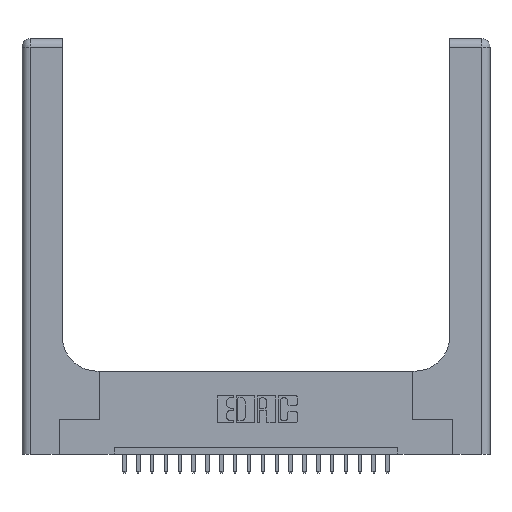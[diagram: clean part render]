
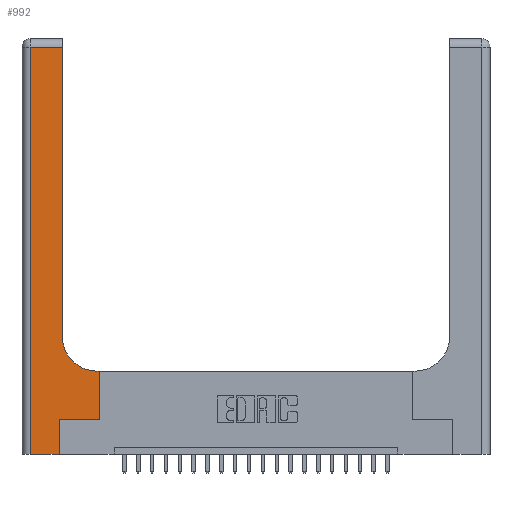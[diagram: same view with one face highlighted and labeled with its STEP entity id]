
A CAD part, top view. The second image highlights one B-rep face of the part: STEP entity #992.
In plain terms, the highlighted planar face has unit normal (0, 0, 1).
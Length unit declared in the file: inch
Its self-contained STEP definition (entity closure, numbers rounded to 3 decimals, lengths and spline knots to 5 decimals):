
#124 = LINE ( 'NONE', #13736, #7437 ) ;
#361 = ORIENTED_EDGE ( 'NONE', *, *, #13297, .T. ) ;
#371 = EDGE_CURVE ( 'NONE', #22887, #6382, #17491, .T. ) ;
#621 = CARTESIAN_POINT ( 'NONE',  ( 0.5585, 0.6, 0.37 ) ) ;
#992 = ADVANCED_FACE ( 'NONE', ( #4005 ), #1167, .F. ) ;
#1020 = EDGE_CURVE ( 'NONE', #8691, #11430, #9333, .T. ) ;
#1040 = DIRECTION ( 'NONE',  ( -1., 0., 0. ) ) ;
#1042 = CARTESIAN_POINT ( 'NONE',  ( 0.269, 0.25, 0.37 ) ) ;
#1167 = PLANE ( 'NONE',  #19967 ) ;
#1243 = VECTOR ( 'NONE', #13216, 39.37008 ) ;
#1485 = CARTESIAN_POINT ( 'NONE',  ( 0.5585, 0.25, 0.37 ) ) ;
#1492 = VECTOR ( 'NONE', #1040, 39.37008 ) ;
#1507 = DIRECTION ( 'NONE',  ( 0., 1., 0. ) ) ;
#1599 = EDGE_CURVE ( 'NONE', #6382, #12002, #2591, .T. ) ;
#1628 = VERTEX_POINT ( 'NONE', #5102 ) ;
#1868 = ORIENTED_EDGE ( 'NONE', *, *, #1020, .T. ) ;
#2591 = LINE ( 'NONE', #19506, #10448 ) ;
#3507 = CARTESIAN_POINT ( 'NONE',  ( 0.5415, 0.85, 0.37 ) ) ;
#4005 = FACE_OUTER_BOUND ( 'NONE', #4035, .T. ) ;
#4035 = EDGE_LOOP ( 'NONE', ( #21562, #4412, #14069, #1868, #361, #22215, #22430, #14792, #4625 ) ) ;
#4412 = ORIENTED_EDGE ( 'NONE', *, *, #15779, .T. ) ;
#4625 = ORIENTED_EDGE ( 'NONE', *, *, #12487, .T. ) ;
#4893 = LINE ( 'NONE', #6259, #1243 ) ;
#5102 = CARTESIAN_POINT ( 'NONE',  ( 0.5415, 0.6, 0.37 ) ) ;
#5917 = LINE ( 'NONE', #19730, #7877 ) ;
#6007 = VECTOR ( 'NONE', #8025, 39.37008 ) ;
#6259 = CARTESIAN_POINT ( 'NONE',  ( 0.269, 0., 0.37 ) ) ;
#6382 = VERTEX_POINT ( 'NONE', #1485 ) ;
#6925 = CIRCLE ( 'NONE', #10398, 0.25 ) ;
#7065 = VERTEX_POINT ( 'NONE', #12906 ) ;
#7305 = CARTESIAN_POINT ( 'NONE',  ( 0.269, 0., 0.37 ) ) ;
#7437 = VECTOR ( 'NONE', #1507, 39.37008 ) ;
#7480 = DIRECTION ( 'NONE',  ( 1., 0., 0. ) ) ;
#7866 = VERTEX_POINT ( 'NONE', #12911 ) ;
#7877 = VECTOR ( 'NONE', #16225, 39.37008 ) ;
#8025 = DIRECTION ( 'NONE',  ( 1., 0., 0. ) ) ;
#8691 = VERTEX_POINT ( 'NONE', #17017 ) ;
#9333 = LINE ( 'NONE', #12786, #12972 ) ;
#9753 = CARTESIAN_POINT ( 'NONE',  ( 0.269, 0.25, 0.37 ) ) ;
#10398 = AXIS2_PLACEMENT_3D ( 'NONE', #3507, #23228, #10555 ) ;
#10448 = VECTOR ( 'NONE', #23183, 39.37008 ) ;
#10555 = DIRECTION ( 'NONE',  ( 1., 0., 0. ) ) ;
#11430 = VERTEX_POINT ( 'NONE', #7305 ) ;
#12002 = VERTEX_POINT ( 'NONE', #621 ) ;
#12487 = EDGE_CURVE ( 'NONE', #1628, #7866, #6925, .T. ) ;
#12786 = CARTESIAN_POINT ( 'NONE',  ( 0., 0., 0.37 ) ) ;
#12906 = CARTESIAN_POINT ( 'NONE',  ( 0.2915, 2.94, 0.37 ) ) ;
#12911 = CARTESIAN_POINT ( 'NONE',  ( 0.2915, 0.85, 0.37 ) ) ;
#12972 = VECTOR ( 'NONE', #7480, 39.37008 ) ;
#13191 = LINE ( 'NONE', #21080, #15462 ) ;
#13216 = DIRECTION ( 'NONE',  ( 0., 1., 0. ) ) ;
#13297 = EDGE_CURVE ( 'NONE', #11430, #22887, #4893, .T. ) ;
#13736 = CARTESIAN_POINT ( 'NONE',  ( 0.2915, 3., 0.37 ) ) ;
#13874 = EDGE_CURVE ( 'NONE', #12002, #1628, #21921, .T. ) ;
#13980 = CARTESIAN_POINT ( 'NONE',  ( 0.06, 2.94, 0.37 ) ) ;
#14069 = ORIENTED_EDGE ( 'NONE', *, *, #16482, .T. ) ;
#14213 = DIRECTION ( 'NONE',  ( -1., 0., 0. ) ) ;
#14698 = DIRECTION ( 'NONE',  ( -1., 0., 0. ) ) ;
#14792 = ORIENTED_EDGE ( 'NONE', *, *, #13874, .T. ) ;
#15462 = VECTOR ( 'NONE', #14213, 39.37008 ) ;
#15779 = EDGE_CURVE ( 'NONE', #7065, #22475, #13191, .T. ) ;
#16225 = DIRECTION ( 'NONE',  ( 0., -1., 0. ) ) ;
#16482 = EDGE_CURVE ( 'NONE', #22475, #8691, #5917, .T. ) ;
#17017 = CARTESIAN_POINT ( 'NONE',  ( 0.06, 0., 0.37 ) ) ;
#17244 = CARTESIAN_POINT ( 'NONE',  ( 0.2915, 0.6, 0.37 ) ) ;
#17491 = LINE ( 'NONE', #9753, #6007 ) ;
#17616 = DIRECTION ( 'NONE',  ( 0., 0., -1. ) ) ;
#19267 = CARTESIAN_POINT ( 'NONE',  ( 0., 3., 0.37 ) ) ;
#19506 = CARTESIAN_POINT ( 'NONE',  ( 0.5585, 0.25, 0.37 ) ) ;
#19730 = CARTESIAN_POINT ( 'NONE',  ( 0.06, 3., 0.37 ) ) ;
#19967 = AXIS2_PLACEMENT_3D ( 'NONE', #19267, #17616, #14698 ) ;
#20062 = EDGE_CURVE ( 'NONE', #7866, #7065, #124, .T. ) ;
#21080 = CARTESIAN_POINT ( 'NONE',  ( 0., 2.94, 0.37 ) ) ;
#21562 = ORIENTED_EDGE ( 'NONE', *, *, #20062, .T. ) ;
#21921 = LINE ( 'NONE', #17244, #1492 ) ;
#22215 = ORIENTED_EDGE ( 'NONE', *, *, #371, .T. ) ;
#22430 = ORIENTED_EDGE ( 'NONE', *, *, #1599, .T. ) ;
#22475 = VERTEX_POINT ( 'NONE', #13980 ) ;
#22887 = VERTEX_POINT ( 'NONE', #1042 ) ;
#23183 = DIRECTION ( 'NONE',  ( 0., 1., 0. ) ) ;
#23228 = DIRECTION ( 'NONE',  ( 0., 0., -1. ) ) ;
